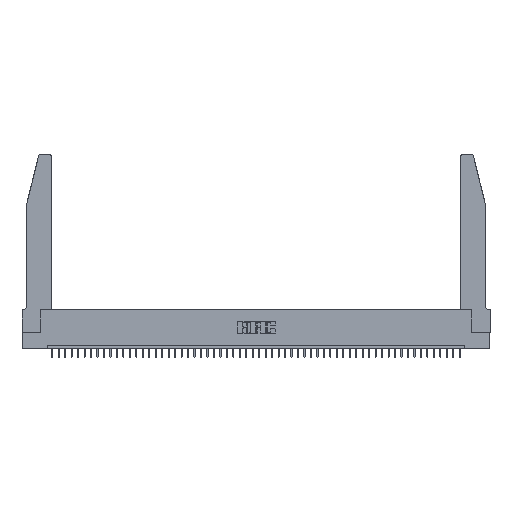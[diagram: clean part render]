
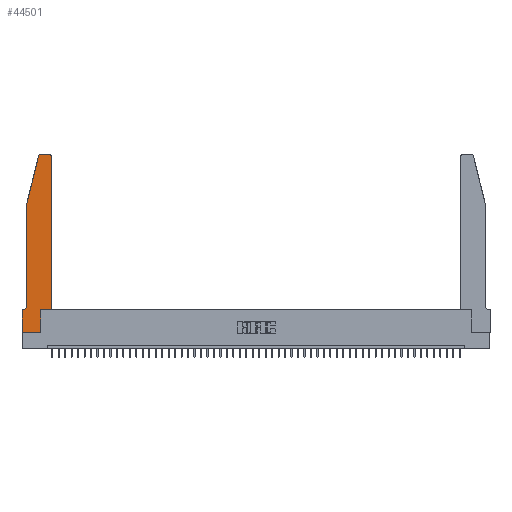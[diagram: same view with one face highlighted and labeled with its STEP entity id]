
A CAD part, top view. The second image highlights one B-rep face of the part: STEP entity #44501.
In plain terms, the highlighted planar face has unit normal (0, 0, 1).
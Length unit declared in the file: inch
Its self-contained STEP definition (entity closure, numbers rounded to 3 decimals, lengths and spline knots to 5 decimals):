
#61 = ORIENTED_EDGE ( 'NONE', *, *, #49171, .T. ) ;
#240 = CARTESIAN_POINT ( 'NONE',  ( 0.0055, 0.35, 0.37 ) ) ;
#2347 = DIRECTION ( 'NONE',  ( 1., 0., 0. ) ) ;
#2708 = CARTESIAN_POINT ( 'NONE',  ( 0.2865, 0., 0.37 ) ) ;
#3707 = CIRCLE ( 'NONE', #19906, 0.03 ) ;
#3937 = DIRECTION ( 'NONE',  ( -1., 0., 0. ) ) ;
#4251 = VERTEX_POINT ( 'NONE', #2708 ) ;
#4288 = LINE ( 'NONE', #45584, #24756 ) ;
#4474 = LINE ( 'NONE', #28322, #20180 ) ;
#5077 = ORIENTED_EDGE ( 'NONE', *, *, #22731, .T. ) ;
#5385 = DIRECTION ( 'NONE',  ( 0., 0., 1. ) ) ;
#5734 = EDGE_CURVE ( 'NONE', #38537, #21601, #4474, .T. ) ;
#5839 = VERTEX_POINT ( 'NONE', #20449 ) ;
#6149 = DIRECTION ( 'NONE',  ( 0., 0., 1. ) ) ;
#6386 = ORIENTED_EDGE ( 'NONE', *, *, #24330, .T. ) ;
#8203 = AXIS2_PLACEMENT_3D ( 'NONE', #10713, #6149, #2347 ) ;
#9039 = DIRECTION ( 'NONE',  ( 0., -1., 0. ) ) ;
#9348 = VERTEX_POINT ( 'NONE', #15666 ) ;
#9449 = CARTESIAN_POINT ( 'NONE',  ( 0.2865, 0.35, 0.37 ) ) ;
#10172 = ORIENTED_EDGE ( 'NONE', *, *, #39298, .T. ) ;
#10713 = CARTESIAN_POINT ( 'NONE',  ( 0., 0.35, 0.37 ) ) ;
#11264 = CARTESIAN_POINT ( 'NONE',  ( 0.2605, 2.75, 0.37 ) ) ;
#11365 = DIRECTION ( 'NONE',  ( -1., 0., 0. ) ) ;
#12732 = VERTEX_POINT ( 'NONE', #240 ) ;
#12982 = CARTESIAN_POINT ( 'NONE',  ( 0.4505, 0.35, 0.37 ) ) ;
#13252 = DIRECTION ( 'NONE',  ( 1., 0., 0. ) ) ;
#13477 = DIRECTION ( 'NONE',  ( 1., 0., 0. ) ) ;
#13537 = VECTOR ( 'NONE', #11365, 39.37008 ) ;
#13771 = PLANE ( 'NONE',  #8203 ) ;
#14425 = VERTEX_POINT ( 'NONE', #42997 ) ;
#14554 = DIRECTION ( 'NONE',  ( -0.239, -0.971, 0. ) ) ;
#15666 = CARTESIAN_POINT ( 'NONE',  ( 0.284, 2.75, 0.37 ) ) ;
#16412 = CARTESIAN_POINT ( 'NONE',  ( 0., 0.35, 0.37 ) ) ;
#17034 = CARTESIAN_POINT ( 'NONE',  ( 0., 0., 0.37 ) ) ;
#17402 = CARTESIAN_POINT ( 'NONE',  ( 0.4505, 0.35, 0.37 ) ) ;
#17534 = EDGE_CURVE ( 'NONE', #21601, #12732, #29340, .T. ) ;
#17687 = VERTEX_POINT ( 'NONE', #28295 ) ;
#18485 = VECTOR ( 'NONE', #39550, 39.37008 ) ;
#18598 = ORIENTED_EDGE ( 'NONE', *, *, #36700, .T. ) ;
#19906 = AXIS2_PLACEMENT_3D ( 'NONE', #45694, #34817, #34574 ) ;
#20180 = VECTOR ( 'NONE', #9039, 39.37008 ) ;
#20449 = CARTESIAN_POINT ( 'NONE',  ( 0.25487, 2.72718, 0.37 ) ) ;
#20603 = LINE ( 'NONE', #9449, #49185 ) ;
#20736 = VECTOR ( 'NONE', #25490, 39.37008 ) ;
#21601 = VERTEX_POINT ( 'NONE', #23115 ) ;
#21753 = ORIENTED_EDGE ( 'NONE', *, *, #36611, .T. ) ;
#22225 = ORIENTED_EDGE ( 'NONE', *, *, #48899, .T. ) ;
#22731 = EDGE_CURVE ( 'NONE', #14425, #4251, #4288, .T. ) ;
#22903 = AXIS2_PLACEMENT_3D ( 'NONE', #44370, #5385, #13252 ) ;
#23115 = CARTESIAN_POINT ( 'NONE',  ( 0.0755, 0.42, 0.37 ) ) ;
#23124 = LINE ( 'NONE', #41843, #23750 ) ;
#23750 = VECTOR ( 'NONE', #14554, 39.37008 ) ;
#24330 = EDGE_CURVE ( 'NONE', #12732, #42006, #45793, .T. ) ;
#24579 = ORIENTED_EDGE ( 'NONE', *, *, #36681, .T. ) ;
#24756 = VECTOR ( 'NONE', #34724, 39.37008 ) ;
#25490 = DIRECTION ( 'NONE',  ( 0., 1., 0. ) ) ;
#28295 = CARTESIAN_POINT ( 'NONE',  ( 0.4505, 2.72, 0.37 ) ) ;
#28322 = CARTESIAN_POINT ( 'NONE',  ( 0.0755, 2., 0.37 ) ) ;
#28694 = ORIENTED_EDGE ( 'NONE', *, *, #46121, .T. ) ;
#29340 = CIRCLE ( 'NONE', #35828, 0.07 ) ;
#30140 = VERTEX_POINT ( 'NONE', #41388 ) ;
#30535 = LINE ( 'NONE', #11264, #34475 ) ;
#30632 = CARTESIAN_POINT ( 'NONE',  ( 0.0755, 0.35, 0.37 ) ) ;
#31732 = ORIENTED_EDGE ( 'NONE', *, *, #17534, .T. ) ;
#33200 = DIRECTION ( 'NONE',  ( 0., 0., -1. ) ) ;
#33293 = VECTOR ( 'NONE', #13477, 39.37008 ) ;
#34475 = VECTOR ( 'NONE', #38337, 39.37008 ) ;
#34574 = DIRECTION ( 'NONE',  ( 1., 0., 0. ) ) ;
#34724 = DIRECTION ( 'NONE',  ( 1., 0., 0. ) ) ;
#34817 = DIRECTION ( 'NONE',  ( 0., 0., 1. ) ) ;
#35277 = VERTEX_POINT ( 'NONE', #39914 ) ;
#35788 = CARTESIAN_POINT ( 'NONE',  ( 0.4505, 0.35, 0.37 ) ) ;
#35828 = AXIS2_PLACEMENT_3D ( 'NONE', #48598, #33200, #3937 ) ;
#36083 = DIRECTION ( 'NONE',  ( 0., 1., 0. ) ) ;
#36611 = EDGE_CURVE ( 'NONE', #37434, #17687, #44704, .T. ) ;
#36681 = EDGE_CURVE ( 'NONE', #35277, #9348, #30535, .T. ) ;
#36700 = EDGE_CURVE ( 'NONE', #9348, #5839, #3707, .T. ) ;
#36872 = EDGE_LOOP ( 'NONE', ( #24579, #18598, #22225, #40382, #31732, #6386, #38015, #5077, #10172, #28694, #21753, #61 ) ) ;
#37434 = VERTEX_POINT ( 'NONE', #12982 ) ;
#38015 = ORIENTED_EDGE ( 'NONE', *, *, #41128, .T. ) ;
#38337 = DIRECTION ( 'NONE',  ( -1., 0., 0. ) ) ;
#38537 = VERTEX_POINT ( 'NONE', #46544 ) ;
#39298 = EDGE_CURVE ( 'NONE', #4251, #30140, #20603, .T. ) ;
#39550 = DIRECTION ( 'NONE',  ( 0., -1., 0. ) ) ;
#39801 = LINE ( 'NONE', #17034, #18485 ) ;
#39914 = CARTESIAN_POINT ( 'NONE',  ( 0.4205, 2.75, 0.37 ) ) ;
#40056 = LINE ( 'NONE', #35788, #33293 ) ;
#40382 = ORIENTED_EDGE ( 'NONE', *, *, #5734, .T. ) ;
#41128 = EDGE_CURVE ( 'NONE', #42006, #14425, #39801, .T. ) ;
#41388 = CARTESIAN_POINT ( 'NONE',  ( 0.2865, 0.35, 0.37 ) ) ;
#41843 = CARTESIAN_POINT ( 'NONE',  ( 0.0755, 2., 0.37 ) ) ;
#42006 = VERTEX_POINT ( 'NONE', #16412 ) ;
#42997 = CARTESIAN_POINT ( 'NONE',  ( 0., 0., 0.37 ) ) ;
#44370 = CARTESIAN_POINT ( 'NONE',  ( 0.4205, 2.72, 0.37 ) ) ;
#44501 = ADVANCED_FACE ( 'NONE', ( #45385 ), #13771, .T. ) ;
#44704 = LINE ( 'NONE', #17402, #20736 ) ;
#44740 = CIRCLE ( 'NONE', #22903, 0.03 ) ;
#45385 = FACE_OUTER_BOUND ( 'NONE', #36872, .T. ) ;
#45584 = CARTESIAN_POINT ( 'NONE',  ( 0., 0., 0.37 ) ) ;
#45694 = CARTESIAN_POINT ( 'NONE',  ( 0.284, 2.72, 0.37 ) ) ;
#45793 = LINE ( 'NONE', #30632, #13537 ) ;
#46121 = EDGE_CURVE ( 'NONE', #30140, #37434, #40056, .T. ) ;
#46544 = CARTESIAN_POINT ( 'NONE',  ( 0.0755, 2., 0.37 ) ) ;
#48598 = CARTESIAN_POINT ( 'NONE',  ( 0.0055, 0.42, 0.37 ) ) ;
#48899 = EDGE_CURVE ( 'NONE', #5839, #38537, #23124, .T. ) ;
#49171 = EDGE_CURVE ( 'NONE', #17687, #35277, #44740, .T. ) ;
#49185 = VECTOR ( 'NONE', #36083, 39.37008 ) ;
